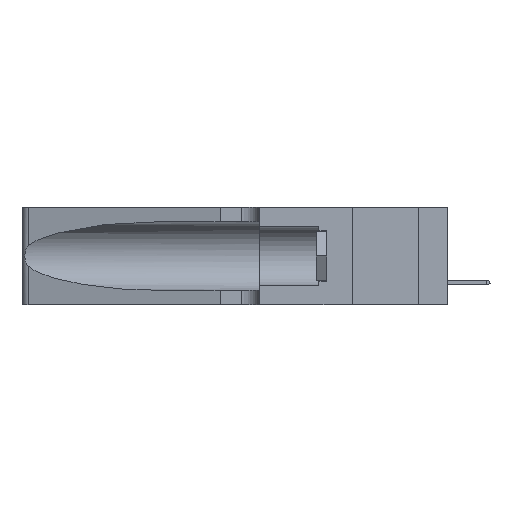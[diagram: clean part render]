
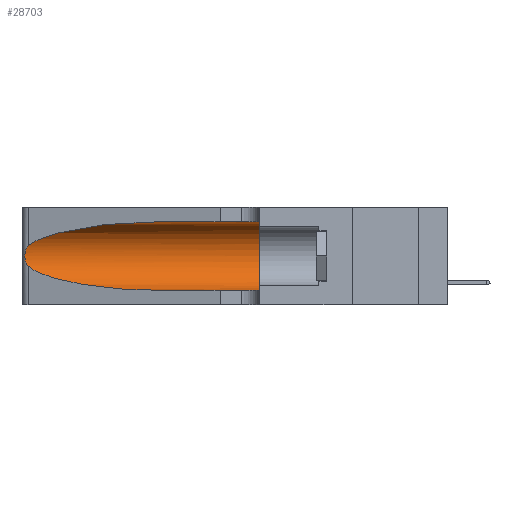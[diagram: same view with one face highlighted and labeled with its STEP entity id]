
A CAD part, left-side view. The second image highlights one B-rep face of the part: STEP entity #28703.
In plain terms, the highlighted cylindrical face has radius 3.308 mm (diameter 6.617 mm), a partial arc.
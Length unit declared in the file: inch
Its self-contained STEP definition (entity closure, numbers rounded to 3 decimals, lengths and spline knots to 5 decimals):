
#1242 = ORIENTED_EDGE ( 'NONE', *, *, #25413, .T. ) ;
#1474 = CARTESIAN_POINT ( 'NONE',  ( 0.1305, 0.72297, 0.05475 ) ) ;
#1890 = CARTESIAN_POINT ( 'NONE',  ( 0.1305, 0.72297, 0.31525 ) ) ;
#1905 = ORIENTED_EDGE ( 'NONE', *, *, #27837, .T. ) ;
#2069 = DIRECTION ( 'NONE',  ( 0., 1., 0. ) ) ;
#2908 = CYLINDRICAL_SURFACE ( 'NONE', #9869, 0.13025 ) ;
#4299 = CARTESIAN_POINT ( 'NONE',  ( 0.1305, 1.61858, 0.31525 ) ) ;
#4986 = ORIENTED_EDGE ( 'NONE', *, *, #42126, .T. ) ;
#5513 = CARTESIAN_POINT ( 'NONE',  ( 0.25487, 1.22718, 0.14631 ) ) ;
#7146 = CARTESIAN_POINT ( 'NONE',  ( 0.25639, 1.23184, 0.21858 ) ) ;
#7677 = CARTESIAN_POINT ( 'NONE',  ( 0.25555, 1.22994, 0.2215 ) ) ;
#8432 = EDGE_LOOP ( 'NONE', ( #4986, #16127, #1242, #1905, #34230, #10117 ) ) ;
#9869 = AXIS2_PLACEMENT_3D ( 'NONE', #44890, #24184, #40491 ) ;
#10117 = ORIENTED_EDGE ( 'NONE', *, *, #20531, .F. ) ;
#11149 = CARTESIAN_POINT ( 'NONE',  ( 0.18966, 0.96281, 0.31525 ) ) ;
#11219 = CARTESIAN_POINT ( 'NONE',  ( 0.25854, 1.2359, 0.20912 ) ) ;
#11392 = CARTESIAN_POINT ( 'NONE',  ( 0.26075, 1.23896, 0.19203 ) ) ;
#12856 = AXIS2_PLACEMENT_3D ( 'NONE', #14855, #2069, #30987 ) ;
#12929 = CARTESIAN_POINT ( 'NONE',  ( 0.1305, 0.72297, 0.05475 ) ) ;
#13102 = CARTESIAN_POINT ( 'NONE',  ( 0.2373, 1.15595, 0.08982 ) ) ;
#14375 = FACE_OUTER_BOUND ( 'NONE', #8432, .T. ) ;
#14659 = CIRCLE ( 'NONE', #12856, 0.13025 ) ;
#14855 = CARTESIAN_POINT ( 'NONE',  ( 0.1305, 0.35, 0.185 ) ) ;
#15332 = CARTESIAN_POINT ( 'NONE',  ( 0.25487, 1.22718, 0.14631 ) ) ;
#16127 = ORIENTED_EDGE ( 'NONE', *, *, #27266, .T. ) ;
#17138 = VERTEX_POINT ( 'NONE', #43265 ) ;
#17184 = VERTEX_POINT ( 'NONE', #39888 ) ;
#19328 = CARTESIAN_POINT ( 'NONE',  ( 0.25487, 1.22718, 0.22369 ) ) ;
#19392 = CARTESIAN_POINT ( 'NONE',  ( 0.25555, 1.22993, 0.14849 ) ) ;
#19953 = CARTESIAN_POINT ( 'NONE',  ( 0.25789, 1.23486, 0.15765 ) ) ;
#20531 = EDGE_CURVE ( 'NONE', #49185, #42941, #39344, .T. ) ;
#22501 = VERTEX_POINT ( 'NONE', #1474 ) ;
#23149 = CARTESIAN_POINT ( 'NONE',  ( 0.1305, 0.35, 0.31525 ) ) ;
#23471 = CARTESIAN_POINT ( 'NONE',  ( 0.25787, 1.23484, 0.2124 ) ) ;
#24184 = DIRECTION ( 'NONE',  ( 0., -1., 0. ) ) ;
#25413 = EDGE_CURVE ( 'NONE', #17138, #22501, #49392, .T. ) ;
#25459 = DIRECTION ( 'NONE',  ( 0., -1., 0. ) ) ;
#27266 = EDGE_CURVE ( 'NONE', #17184, #17138, #51032, .T. ) ;
#27457 = CARTESIAN_POINT ( 'NONE',  ( 0.1305, 0.72297, 0.31525 ) ) ;
#27837 = EDGE_CURVE ( 'NONE', #22501, #43706, #30287, .T. ) ;
#28703 = ADVANCED_FACE ( 'NONE', ( #14375 ), #2908, .F. ) ;
#29057 = DIRECTION ( 'NONE',  ( 0., -1., 0. ) ) ;
#30287 = LINE ( 'NONE', #45679, #38573 ) ;
#30987 = DIRECTION ( 'NONE',  ( 0., 0., 1. ) ) ;
#33465 = CARTESIAN_POINT ( 'NONE',  ( 0.18966, 0.96281, 0.05475 ) ) ;
#34230 = ORIENTED_EDGE ( 'NONE', *, *, #51230, .F. ) ;
#35834 = CARTESIAN_POINT ( 'NONE',  ( 0.26075, 1.23896, 0.178 ) ) ;
#36675 = CARTESIAN_POINT ( 'NONE',  ( 0.1305, 0.35, 0.05475 ) ) ;
#38573 = VECTOR ( 'NONE', #25459, 39.37008 ) ;
#38984 = CARTESIAN_POINT ( 'NONE',  ( 0.2373, 1.15595, 0.28018 ) ) ;
#39344 = LINE ( 'NONE', #4299, #42475 ) ;
#39571 = CARTESIAN_POINT ( 'NONE',  ( 0.26018, 1.23835, 0.19895 ) ) ;
#39888 = CARTESIAN_POINT ( 'NONE',  ( 0.25487, 1.22718, 0.22369 ) ) ;
#39958 = CARTESIAN_POINT ( 'NONE',  ( 0.26017, 1.23833, 0.17102 ) ) ;
#40299 = CARTESIAN_POINT ( 'NONE',  ( 0.25487, 1.22718, 0.22369 ) ) ;
#40491 = DIRECTION ( 'NONE',  ( 0., 0., -1. ) ) ;
#42126 = EDGE_CURVE ( 'NONE', #49185, #17184, #51365, .T. ) ;
#42475 = VECTOR ( 'NONE', #29057, 39.37008 ) ;
#42941 = VERTEX_POINT ( 'NONE', #23149 ) ;
#43265 = CARTESIAN_POINT ( 'NONE',  ( 0.25487, 1.22718, 0.14631 ) ) ;
#43706 = VERTEX_POINT ( 'NONE', #36675 ) ;
#44028 = CARTESIAN_POINT ( 'NONE',  ( 0.25856, 1.23593, 0.16098 ) ) ;
#44372 = CARTESIAN_POINT ( 'NONE',  ( 0.25639, 1.23186, 0.15144 ) ) ;
#44890 = CARTESIAN_POINT ( 'NONE',  ( 0.1305, 1.61858, 0.185 ) ) ;
#45679 = CARTESIAN_POINT ( 'NONE',  ( 0.1305, 1.61858, 0.05475 ) ) ;
#49185 = VERTEX_POINT ( 'NONE', #27457 ) ;
#49392 =( BOUNDED_CURVE ( )  B_SPLINE_CURVE ( 3, ( #5513, #13102, #33465, #12929 ),
 .UNSPECIFIED., .F., .F. ) 
 B_SPLINE_CURVE_WITH_KNOTS ( ( 4, 4 ),
 ( 3.44316, 4.71239 ),
 .UNSPECIFIED. ) 
 CURVE ( )  GEOMETRIC_REPRESENTATION_ITEM ( )  RATIONAL_B_SPLINE_CURVE ( ( 1., 0.87, 0.87, 1. ) ) 
 REPRESENTATION_ITEM ( '' )  );
#51032 = B_SPLINE_CURVE_WITH_KNOTS ( 'NONE', 3,
 ( #40299, #7677, #7146, #23471, #11219, #39571, #11392, #35834, #39958, #44028, #19953, #44372, #19392, #15332 ),
 .UNSPECIFIED., .F., .F.,
 ( 4, 2, 2, 2, 2, 2, 4 ),
 ( 0., 0.00027, 0.00053, 0.00107, 0.0016, 0.00187, 0.00214 ),
 .UNSPECIFIED. ) ;
#51230 = EDGE_CURVE ( 'NONE', #42941, #43706, #14659, .T. ) ;
#51365 =( BOUNDED_CURVE ( )  B_SPLINE_CURVE ( 3, ( #1890, #11149, #38984, #19328 ),
 .UNSPECIFIED., .F., .T. ) 
 B_SPLINE_CURVE_WITH_KNOTS ( ( 4, 4 ),
 ( 1.5708, 2.84003 ),
 .UNSPECIFIED. ) 
 CURVE ( )  GEOMETRIC_REPRESENTATION_ITEM ( )  RATIONAL_B_SPLINE_CURVE ( ( 1., 0.87, 0.87, 1. ) ) 
 REPRESENTATION_ITEM ( '' )  );
